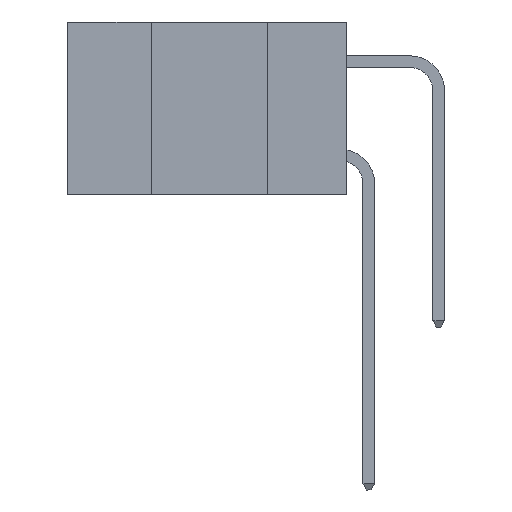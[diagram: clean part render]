
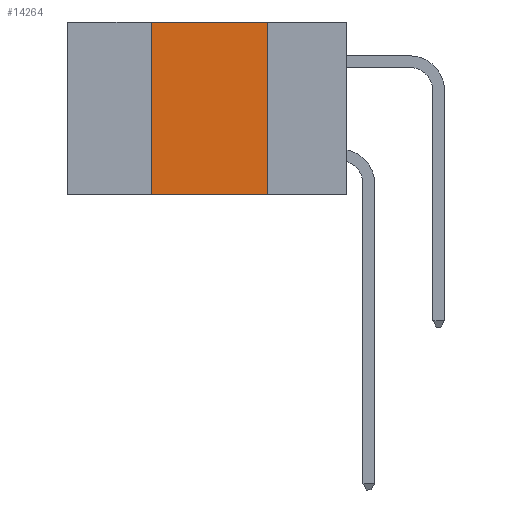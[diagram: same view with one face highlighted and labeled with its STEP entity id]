
A CAD part, left-side view. The second image highlights one B-rep face of the part: STEP entity #14264.
In plain terms, the highlighted planar face has unit normal (-1, 0, 0).
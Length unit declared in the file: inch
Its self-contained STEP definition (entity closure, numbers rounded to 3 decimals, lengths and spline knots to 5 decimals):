
#833 = CARTESIAN_POINT ( 'NONE',  ( 0., 0.42, 0. ) ) ;
#937 = VERTEX_POINT ( 'NONE', #833 ) ;
#2013 = VERTEX_POINT ( 'NONE', #18659 ) ;
#2573 = CARTESIAN_POINT ( 'NONE',  ( 0., 0.6, 0. ) ) ;
#2915 = CARTESIAN_POINT ( 'NONE',  ( 0., 0.17, 0. ) ) ;
#3546 = DIRECTION ( 'NONE',  ( 0., -1., 0. ) ) ;
#3869 = LINE ( 'NONE', #20062, #14117 ) ;
#4100 = VECTOR ( 'NONE', #20248, 39.37008 ) ;
#4406 = DIRECTION ( 'NONE',  ( 1., 0., 0. ) ) ;
#5225 = ORIENTED_EDGE ( 'NONE', *, *, #16638, .F. ) ;
#5375 = ORIENTED_EDGE ( 'NONE', *, *, #17347, .F. ) ;
#5805 = AXIS2_PLACEMENT_3D ( 'NONE', #2573, #4406, #16479 ) ;
#5877 = FACE_OUTER_BOUND ( 'NONE', #9837, .T. ) ;
#6153 = CARTESIAN_POINT ( 'NONE',  ( 0., 0.42, -0.37 ) ) ;
#7758 = CARTESIAN_POINT ( 'NONE',  ( 0., 0.17, 0. ) ) ;
#8476 = VERTEX_POINT ( 'NONE', #6153 ) ;
#8681 = LINE ( 'NONE', #2915, #4100 ) ;
#9837 = EDGE_LOOP ( 'NONE', ( #19089, #5225, #5375, #17338 ) ) ;
#11158 = VERTEX_POINT ( 'NONE', #7758 ) ;
#12517 = VECTOR ( 'NONE', #21904, 39.37008 ) ;
#12688 = EDGE_CURVE ( 'NONE', #8476, #2013, #13795, .T. ) ;
#13795 = LINE ( 'NONE', #13883, #19499 ) ;
#13883 = CARTESIAN_POINT ( 'NONE',  ( 0., 0.6, -0.37 ) ) ;
#14117 = VECTOR ( 'NONE', #16605, 39.37008 ) ;
#14264 = ADVANCED_FACE ( 'NONE', ( #5877 ), #19869, .F. ) ;
#16479 = DIRECTION ( 'NONE',  ( 0., 0., -1. ) ) ;
#16605 = DIRECTION ( 'NONE',  ( 0., -1., 0. ) ) ;
#16638 = EDGE_CURVE ( 'NONE', #937, #11158, #3869, .T. ) ;
#17338 = ORIENTED_EDGE ( 'NONE', *, *, #12688, .T. ) ;
#17347 = EDGE_CURVE ( 'NONE', #8476, #937, #21598, .T. ) ;
#18492 = EDGE_CURVE ( 'NONE', #11158, #2013, #8681, .T. ) ;
#18659 = CARTESIAN_POINT ( 'NONE',  ( 0., 0.17, -0.37 ) ) ;
#19089 = ORIENTED_EDGE ( 'NONE', *, *, #18492, .F. ) ;
#19499 = VECTOR ( 'NONE', #3546, 39.37008 ) ;
#19869 = PLANE ( 'NONE',  #5805 ) ;
#20062 = CARTESIAN_POINT ( 'NONE',  ( 0., 0.6, 0. ) ) ;
#20248 = DIRECTION ( 'NONE',  ( 0., 0., -1. ) ) ;
#21598 = LINE ( 'NONE', #21832, #12517 ) ;
#21832 = CARTESIAN_POINT ( 'NONE',  ( 0., 0.42, 0. ) ) ;
#21904 = DIRECTION ( 'NONE',  ( 0., 0., 1. ) ) ;
